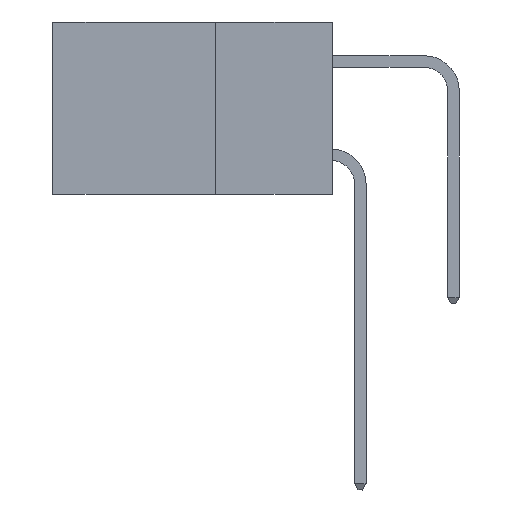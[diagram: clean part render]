
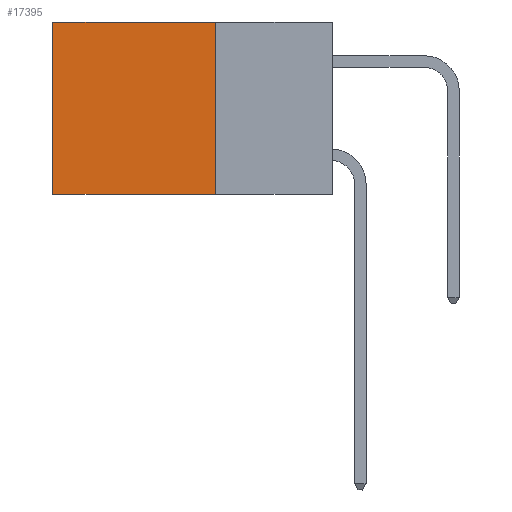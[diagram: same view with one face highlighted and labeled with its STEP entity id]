
A CAD part, left-side view. The second image highlights one B-rep face of the part: STEP entity #17395.
In plain terms, the highlighted planar face has unit normal (-1, 0, 0).
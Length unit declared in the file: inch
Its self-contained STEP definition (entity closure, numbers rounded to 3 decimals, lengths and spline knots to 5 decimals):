
#312 = EDGE_CURVE ( 'NONE', #15844, #6328, #17201, .T. ) ;
#1020 = DIRECTION ( 'NONE',  ( 0., 0., -1. ) ) ;
#1106 = DIRECTION ( 'NONE',  ( 0., 0., -1. ) ) ;
#2883 = ORIENTED_EDGE ( 'NONE', *, *, #3718, .T. ) ;
#3206 = DIRECTION ( 'NONE',  ( 0., 1., 0. ) ) ;
#3496 = CARTESIAN_POINT ( 'NONE',  ( 0.298, 0.6, -0.37 ) ) ;
#3718 = EDGE_CURVE ( 'NONE', #6328, #7151, #14846, .T. ) ;
#4660 = PLANE ( 'NONE',  #7661 ) ;
#5811 = ORIENTED_EDGE ( 'NONE', *, *, #15505, .F. ) ;
#6328 = VERTEX_POINT ( 'NONE', #20849 ) ;
#6636 = CARTESIAN_POINT ( 'NONE',  ( 0.298, 0.25, 0. ) ) ;
#7151 = VERTEX_POINT ( 'NONE', #3496 ) ;
#7661 = AXIS2_PLACEMENT_3D ( 'NONE', #9793, #18044, #1106 ) ;
#8770 = DIRECTION ( 'NONE',  ( 0., 1., 0. ) ) ;
#9476 = ORIENTED_EDGE ( 'NONE', *, *, #18090, .F. ) ;
#9793 = CARTESIAN_POINT ( 'NONE',  ( 0.298, 0.25, 0. ) ) ;
#10172 = LINE ( 'NONE', #19265, #20566 ) ;
#11664 = CARTESIAN_POINT ( 'NONE',  ( 0.298, 0.25, 0. ) ) ;
#11675 = VECTOR ( 'NONE', #1020, 39.37008 ) ;
#11794 = FACE_OUTER_BOUND ( 'NONE', #12058, .T. ) ;
#11810 = VECTOR ( 'NONE', #3206, 39.37008 ) ;
#12058 = EDGE_LOOP ( 'NONE', ( #2883, #5811, #9476, #19914 ) ) ;
#14846 = LINE ( 'NONE', #17652, #11675 ) ;
#15505 = EDGE_CURVE ( 'NONE', #17438, #7151, #21430, .T. ) ;
#15844 = VERTEX_POINT ( 'NONE', #6636 ) ;
#15983 = DIRECTION ( 'NONE',  ( 0., 0., -1. ) ) ;
#16774 = CARTESIAN_POINT ( 'NONE',  ( 0.298, 0.25, -0.37 ) ) ;
#17201 = LINE ( 'NONE', #11664, #21765 ) ;
#17395 = ADVANCED_FACE ( 'NONE', ( #11794 ), #4660, .F. ) ;
#17438 = VERTEX_POINT ( 'NONE', #21611 ) ;
#17652 = CARTESIAN_POINT ( 'NONE',  ( 0.298, 0.6, 0. ) ) ;
#18044 = DIRECTION ( 'NONE',  ( 1., 0., 0. ) ) ;
#18090 = EDGE_CURVE ( 'NONE', #15844, #17438, #10172, .T. ) ;
#19265 = CARTESIAN_POINT ( 'NONE',  ( 0.298, 0.25, 0. ) ) ;
#19914 = ORIENTED_EDGE ( 'NONE', *, *, #312, .T. ) ;
#20566 = VECTOR ( 'NONE', #15983, 39.37008 ) ;
#20849 = CARTESIAN_POINT ( 'NONE',  ( 0.298, 0.6, 0. ) ) ;
#21430 = LINE ( 'NONE', #16774, #11810 ) ;
#21611 = CARTESIAN_POINT ( 'NONE',  ( 0.298, 0.25, -0.37 ) ) ;
#21765 = VECTOR ( 'NONE', #8770, 39.37008 ) ;
